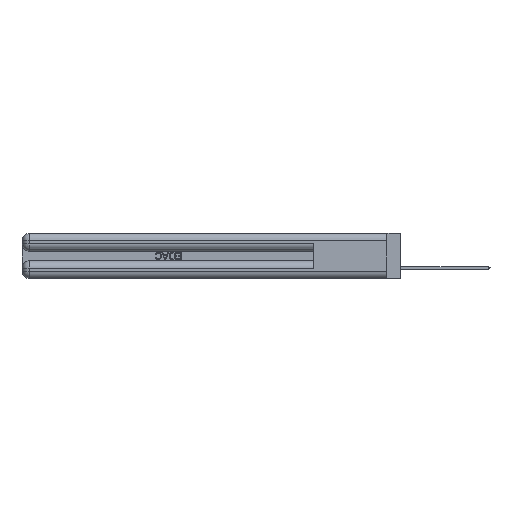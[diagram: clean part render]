
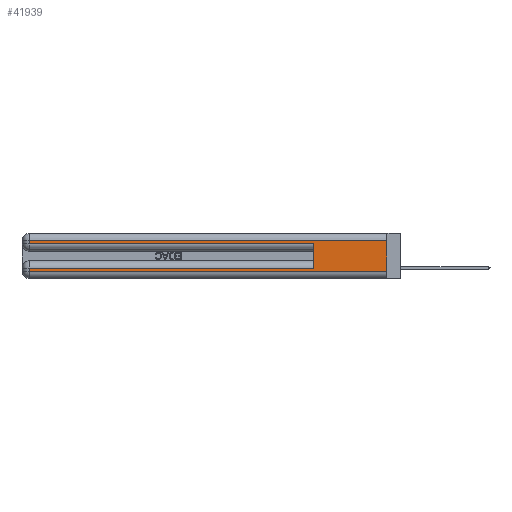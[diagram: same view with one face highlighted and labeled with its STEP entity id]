
A CAD part, left-side view. The second image highlights one B-rep face of the part: STEP entity #41939.
In plain terms, the highlighted planar face has unit normal (-1, 0, 0).
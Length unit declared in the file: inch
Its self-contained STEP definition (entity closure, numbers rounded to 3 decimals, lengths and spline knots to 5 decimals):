
#659 = DIRECTION ( 'NONE',  ( 0., 0., 1. ) ) ;
#676 = EDGE_CURVE ( 'NONE', #48017, #37138, #16700, .T. ) ;
#897 = LINE ( 'NONE', #40906, #4823 ) ;
#1230 = DIRECTION ( 'NONE',  ( 0., 1., 0. ) ) ;
#2540 = LINE ( 'NONE', #5706, #34447 ) ;
#3893 = LINE ( 'NONE', #31185, #42308 ) ;
#4823 = VECTOR ( 'NONE', #13309, 39.37008 ) ;
#5706 = CARTESIAN_POINT ( 'NONE',  ( 0., 0.6, 0.145 ) ) ;
#5825 = CARTESIAN_POINT ( 'NONE',  ( 0., 0., 0.37 ) ) ;
#5997 = VECTOR ( 'NONE', #1230, 39.37008 ) ;
#6712 = ORIENTED_EDGE ( 'NONE', *, *, #30256, .F. ) ;
#8622 = LINE ( 'NONE', #34245, #5997 ) ;
#11791 = DIRECTION ( 'NONE',  ( 1., 0., 0. ) ) ;
#13309 = DIRECTION ( 'NONE',  ( 0., 0., -1. ) ) ;
#13473 = FACE_OUTER_BOUND ( 'NONE', #53862, .T. ) ;
#14804 = CARTESIAN_POINT ( 'NONE',  ( 0., 2.94, 0.085 ) ) ;
#16700 = LINE ( 'NONE', #26926, #49911 ) ;
#16996 = DIRECTION ( 'NONE',  ( 0., 0., -1. ) ) ;
#19740 = VERTEX_POINT ( 'NONE', #14804 ) ;
#20720 = CARTESIAN_POINT ( 'NONE',  ( 0., 0., 0.37 ) ) ;
#24038 = PLANE ( 'NONE',  #46761 ) ;
#24516 = CARTESIAN_POINT ( 'NONE',  ( 0., 2.94, 0.37 ) ) ;
#26926 = CARTESIAN_POINT ( 'NONE',  ( 0., 0., 0.31 ) ) ;
#28198 = ORIENTED_EDGE ( 'NONE', *, *, #38563, .T. ) ;
#29765 = EDGE_CURVE ( 'NONE', #45409, #45697, #3893, .T. ) ;
#30256 = EDGE_CURVE ( 'NONE', #35075, #51724, #2540, .T. ) ;
#31185 = CARTESIAN_POINT ( 'NONE',  ( 0., 0., 0.06 ) ) ;
#31268 = DIRECTION ( 'NONE',  ( 0., 1., 0. ) ) ;
#32364 = ORIENTED_EDGE ( 'NONE', *, *, #48641, .F. ) ;
#32731 = DIRECTION ( 'NONE',  ( 0., -1., 0. ) ) ;
#32905 = CARTESIAN_POINT ( 'NONE',  ( 0., 0., 0.285 ) ) ;
#33298 = CARTESIAN_POINT ( 'NONE',  ( 0., 0., 0.31 ) ) ;
#34245 = CARTESIAN_POINT ( 'NONE',  ( 0., 0., 0.085 ) ) ;
#34447 = VECTOR ( 'NONE', #659, 39.37008 ) ;
#34570 = CARTESIAN_POINT ( 'NONE',  ( 0., 0.6, 0.285 ) ) ;
#34908 = VECTOR ( 'NONE', #16996, 39.37008 ) ;
#35075 = VERTEX_POINT ( 'NONE', #44591 ) ;
#35429 = EDGE_CURVE ( 'NONE', #44345, #51724, #51460, .T. ) ;
#35763 = CARTESIAN_POINT ( 'NONE',  ( 0., 2.94, 0.31 ) ) ;
#36944 = DIRECTION ( 'NONE',  ( 0., 0., -1. ) ) ;
#37138 = VERTEX_POINT ( 'NONE', #35763 ) ;
#37992 = ORIENTED_EDGE ( 'NONE', *, *, #676, .T. ) ;
#38563 = EDGE_CURVE ( 'NONE', #35075, #19740, #8622, .T. ) ;
#38626 = DIRECTION ( 'NONE',  ( 0., 0., -1. ) ) ;
#40770 = ORIENTED_EDGE ( 'NONE', *, *, #29765, .T. ) ;
#40906 = CARTESIAN_POINT ( 'NONE',  ( 0., 2.94, 0.37 ) ) ;
#41188 = CARTESIAN_POINT ( 'NONE',  ( 0., 2.94, 0.06 ) ) ;
#41939 = ADVANCED_FACE ( 'NONE', ( #13473 ), #24038, .F. ) ;
#42308 = VECTOR ( 'NONE', #47546, 39.37008 ) ;
#42437 = VECTOR ( 'NONE', #38626, 39.37008 ) ;
#43747 = LINE ( 'NONE', #5825, #42437 ) ;
#43781 = EDGE_CURVE ( 'NONE', #37138, #44345, #897, .T. ) ;
#44345 = VERTEX_POINT ( 'NONE', #52803 ) ;
#44591 = CARTESIAN_POINT ( 'NONE',  ( 0., 0.6, 0.085 ) ) ;
#45409 = VERTEX_POINT ( 'NONE', #41188 ) ;
#45697 = VERTEX_POINT ( 'NONE', #45723 ) ;
#45723 = CARTESIAN_POINT ( 'NONE',  ( 0., 0., 0.06 ) ) ;
#46015 = ORIENTED_EDGE ( 'NONE', *, *, #35429, .T. ) ;
#46761 = AXIS2_PLACEMENT_3D ( 'NONE', #20720, #11791, #36944 ) ;
#46912 = ORIENTED_EDGE ( 'NONE', *, *, #43781, .T. ) ;
#47546 = DIRECTION ( 'NONE',  ( 0., -1., 0. ) ) ;
#48017 = VERTEX_POINT ( 'NONE', #33298 ) ;
#48202 = VECTOR ( 'NONE', #32731, 39.37008 ) ;
#48641 = EDGE_CURVE ( 'NONE', #48017, #45697, #43747, .T. ) ;
#49911 = VECTOR ( 'NONE', #31268, 39.37008 ) ;
#50041 = ORIENTED_EDGE ( 'NONE', *, *, #52727, .T. ) ;
#51460 = LINE ( 'NONE', #32905, #48202 ) ;
#51724 = VERTEX_POINT ( 'NONE', #34570 ) ;
#51866 = LINE ( 'NONE', #24516, #34908 ) ;
#52727 = EDGE_CURVE ( 'NONE', #19740, #45409, #51866, .T. ) ;
#52803 = CARTESIAN_POINT ( 'NONE',  ( 0., 2.94, 0.285 ) ) ;
#53862 = EDGE_LOOP ( 'NONE', ( #32364, #37992, #46912, #46015, #6712, #28198, #50041, #40770 ) ) ;
